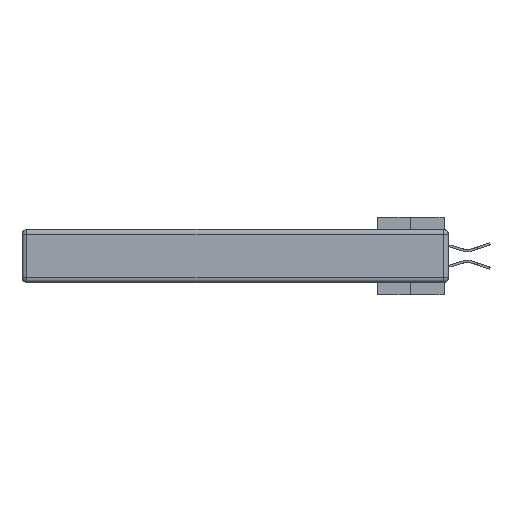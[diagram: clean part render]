
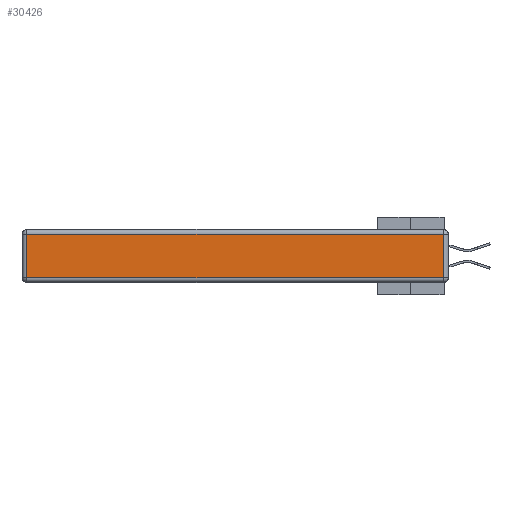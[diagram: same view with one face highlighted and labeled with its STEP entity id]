
A CAD part, left-side view. The second image highlights one B-rep face of the part: STEP entity #30426.
In plain terms, the highlighted planar face has unit normal (-1, 0, 0).
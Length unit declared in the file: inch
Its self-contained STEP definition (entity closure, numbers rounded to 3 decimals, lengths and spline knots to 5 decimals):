
#299 = EDGE_CURVE ( 'NONE', #4494, #19873, #5608, .T. ) ;
#2832 = DIRECTION ( 'NONE',  ( 0., 0., -1. ) ) ;
#3564 = CARTESIAN_POINT ( 'NONE',  ( 0., 0.03, -0.343 ) ) ;
#4494 = VERTEX_POINT ( 'NONE', #31880 ) ;
#5161 = VERTEX_POINT ( 'NONE', #19945 ) ;
#5608 = LINE ( 'NONE', #3564, #17762 ) ;
#5701 = EDGE_CURVE ( 'NONE', #19873, #5161, #21699, .T. ) ;
#5813 = LINE ( 'NONE', #14907, #33869 ) ;
#7627 = DIRECTION ( 'NONE',  ( 0., 1., 0. ) ) ;
#9138 = VERTEX_POINT ( 'NONE', #30572 ) ;
#9581 = DIRECTION ( 'NONE',  ( 0., 0., 1. ) ) ;
#10526 = VECTOR ( 'NONE', #19446, 39.37008 ) ;
#14907 = CARTESIAN_POINT ( 'NONE',  ( 0., 2.72, -0.343 ) ) ;
#15114 = ORIENTED_EDGE ( 'NONE', *, *, #5701, .T. ) ;
#16075 = AXIS2_PLACEMENT_3D ( 'NONE', #28103, #18939, #9581 ) ;
#16649 = EDGE_CURVE ( 'NONE', #5161, #9138, #5813, .T. ) ;
#17762 = VECTOR ( 'NONE', #31053, 39.37008 ) ;
#18561 = EDGE_CURVE ( 'NONE', #9138, #4494, #22151, .T. ) ;
#18939 = DIRECTION ( 'NONE',  ( -1., 0., 0. ) ) ;
#19312 = PLANE ( 'NONE',  #16075 ) ;
#19446 = DIRECTION ( 'NONE',  ( 0., -1., 0. ) ) ;
#19873 = VERTEX_POINT ( 'NONE', #25197 ) ;
#19945 = CARTESIAN_POINT ( 'NONE',  ( 0., 2.72, -0.03 ) ) ;
#21165 = ORIENTED_EDGE ( 'NONE', *, *, #299, .T. ) ;
#21699 = LINE ( 'NONE', #35414, #28504 ) ;
#22151 = LINE ( 'NONE', #29066, #10526 ) ;
#25197 = CARTESIAN_POINT ( 'NONE',  ( 0., 0.03, -0.03 ) ) ;
#28103 = CARTESIAN_POINT ( 'NONE',  ( 0., 0., -0.343 ) ) ;
#28389 = FACE_OUTER_BOUND ( 'NONE', #30546, .T. ) ;
#28504 = VECTOR ( 'NONE', #7627, 39.37008 ) ;
#29066 = CARTESIAN_POINT ( 'NONE',  ( 0., 0., -0.313 ) ) ;
#30426 = ADVANCED_FACE ( 'NONE', ( #28389 ), #19312, .T. ) ;
#30546 = EDGE_LOOP ( 'NONE', ( #39901, #21165, #15114, #36994 ) ) ;
#30572 = CARTESIAN_POINT ( 'NONE',  ( 0., 2.72, -0.313 ) ) ;
#31053 = DIRECTION ( 'NONE',  ( 0., 0., 1. ) ) ;
#31880 = CARTESIAN_POINT ( 'NONE',  ( 0., 0.03, -0.313 ) ) ;
#33869 = VECTOR ( 'NONE', #2832, 39.37008 ) ;
#35414 = CARTESIAN_POINT ( 'NONE',  ( 0., 2.75, -0.03 ) ) ;
#36994 = ORIENTED_EDGE ( 'NONE', *, *, #16649, .T. ) ;
#39901 = ORIENTED_EDGE ( 'NONE', *, *, #18561, .T. ) ;
